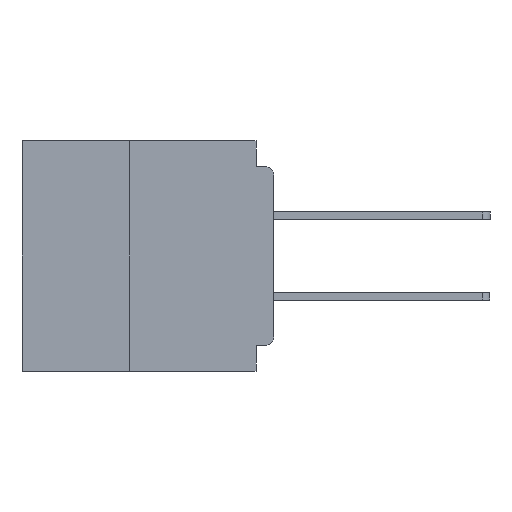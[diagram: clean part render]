
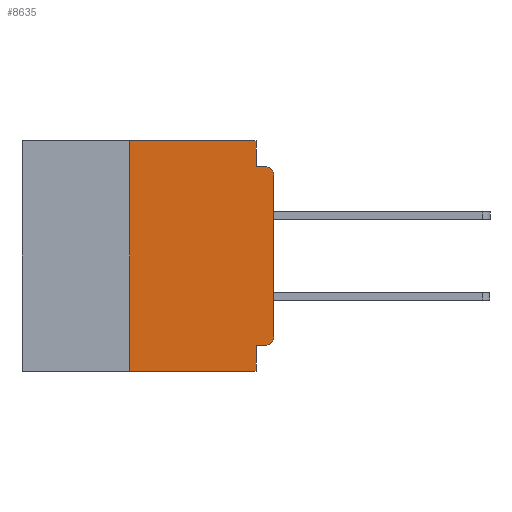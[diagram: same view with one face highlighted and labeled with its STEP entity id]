
A CAD part, left-side view. The second image highlights one B-rep face of the part: STEP entity #8635.
In plain terms, the highlighted planar face has unit normal (-1, 0, 0).
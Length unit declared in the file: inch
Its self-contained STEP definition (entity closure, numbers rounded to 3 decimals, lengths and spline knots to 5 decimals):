
#691 = CARTESIAN_POINT ( 'NONE',  ( 0., 0.031, 0. ) ) ;
#788 = CIRCLE ( 'NONE', #22357, 0.015 ) ;
#1027 = CARTESIAN_POINT ( 'NONE',  ( 0., 0.437, 0. ) ) ;
#2034 = CARTESIAN_POINT ( 'NONE',  ( 0., 0.015, -0.045 ) ) ;
#2985 = EDGE_CURVE ( 'NONE', #43031, #33308, #5848, .T. ) ;
#2990 = LINE ( 'NONE', #50538, #21661 ) ;
#3329 = CARTESIAN_POINT ( 'NONE',  ( 0., 0.015, -0.06 ) ) ;
#5081 = EDGE_CURVE ( 'NONE', #33308, #11062, #788, .T. ) ;
#5328 = EDGE_CURVE ( 'NONE', #40822, #6536, #53416, .T. ) ;
#5631 = VERTEX_POINT ( 'NONE', #53256 ) ;
#5848 = LINE ( 'NONE', #26237, #15844 ) ;
#6536 = VERTEX_POINT ( 'NONE', #42784 ) ;
#7572 = DIRECTION ( 'NONE',  ( 0., 0., -1. ) ) ;
#8548 = ORIENTED_EDGE ( 'NONE', *, *, #28978, .T. ) ;
#8635 = ADVANCED_FACE ( 'NONE', ( #8976 ), #18009, .F. ) ;
#8976 = FACE_OUTER_BOUND ( 'NONE', #48252, .T. ) ;
#9121 = VECTOR ( 'NONE', #34811, 39.37008 ) ;
#9274 = VERTEX_POINT ( 'NONE', #18303 ) ;
#9562 = DIRECTION ( 'NONE',  ( 0., 0., -1. ) ) ;
#10296 = CARTESIAN_POINT ( 'NONE',  ( 0., 0., -0.06 ) ) ;
#11062 = VERTEX_POINT ( 'NONE', #2034 ) ;
#11220 = CARTESIAN_POINT ( 'NONE',  ( 0., 0.437, -0.4 ) ) ;
#12491 = LINE ( 'NONE', #11220, #33768 ) ;
#12582 = LINE ( 'NONE', #50322, #36496 ) ;
#13017 = VECTOR ( 'NONE', #22300, 39.37008 ) ;
#13516 = DIRECTION ( 'NONE',  ( 0., 0., 1. ) ) ;
#15212 = ORIENTED_EDGE ( 'NONE', *, *, #45005, .F. ) ;
#15306 = AXIS2_PLACEMENT_3D ( 'NONE', #1027, #35007, #9562 ) ;
#15700 = LINE ( 'NONE', #43263, #13017 ) ;
#15844 = VECTOR ( 'NONE', #26542, 39.37008 ) ;
#15847 = VERTEX_POINT ( 'NONE', #26275 ) ;
#17436 = VERTEX_POINT ( 'NONE', #44645 ) ;
#18009 = PLANE ( 'NONE',  #15306 ) ;
#18303 = CARTESIAN_POINT ( 'NONE',  ( 0., 0.031, -0.045 ) ) ;
#18527 = CARTESIAN_POINT ( 'NONE',  ( 0., 0.015, -0.34 ) ) ;
#19420 = EDGE_CURVE ( 'NONE', #15847, #17436, #21858, .T. ) ;
#20722 = EDGE_CURVE ( 'NONE', #17436, #5631, #15700, .T. ) ;
#21186 = EDGE_CURVE ( 'NONE', #9274, #11062, #2990, .T. ) ;
#21661 = VECTOR ( 'NONE', #34069, 39.37008 ) ;
#21858 = LINE ( 'NONE', #22060, #9121 ) ;
#21923 = ORIENTED_EDGE ( 'NONE', *, *, #5328, .F. ) ;
#22060 = CARTESIAN_POINT ( 'NONE',  ( 0., 0., -0.355 ) ) ;
#22300 = DIRECTION ( 'NONE',  ( 0., 0., -1. ) ) ;
#22357 = AXIS2_PLACEMENT_3D ( 'NONE', #3329, #33064, #7572 ) ;
#22798 = DIRECTION ( 'NONE',  ( 0., 0., -1. ) ) ;
#25472 = CARTESIAN_POINT ( 'NONE',  ( 0., 0.031, 0. ) ) ;
#25900 = ORIENTED_EDGE ( 'NONE', *, *, #43284, .T. ) ;
#26237 = CARTESIAN_POINT ( 'NONE',  ( 0., 0., 0. ) ) ;
#26275 = CARTESIAN_POINT ( 'NONE',  ( 0., 0.015, -0.355 ) ) ;
#26542 = DIRECTION ( 'NONE',  ( 0., 0., 1. ) ) ;
#28978 = EDGE_CURVE ( 'NONE', #15847, #43031, #40897, .T. ) ;
#29387 = EDGE_CURVE ( 'NONE', #6536, #44907, #12582, .T. ) ;
#30440 = CARTESIAN_POINT ( 'NONE',  ( 0., 0.25, -0.4 ) ) ;
#30451 = DIRECTION ( 'NONE',  ( 0., 0., -1. ) ) ;
#33064 = DIRECTION ( 'NONE',  ( -1., 0., 0. ) ) ;
#33308 = VERTEX_POINT ( 'NONE', #10296 ) ;
#33573 = VECTOR ( 'NONE', #30451, 39.37008 ) ;
#33768 = VECTOR ( 'NONE', #36654, 39.37008 ) ;
#34069 = DIRECTION ( 'NONE',  ( 0., -1., 0. ) ) ;
#34811 = DIRECTION ( 'NONE',  ( 0., 1., 0. ) ) ;
#35007 = DIRECTION ( 'NONE',  ( 1., 0., 0. ) ) ;
#36496 = VECTOR ( 'NONE', #54429, 39.37008 ) ;
#36654 = DIRECTION ( 'NONE',  ( 0., -1., 0. ) ) ;
#40822 = VERTEX_POINT ( 'NONE', #44961 ) ;
#40897 = CIRCLE ( 'NONE', #43734, 0.015 ) ;
#42530 = VECTOR ( 'NONE', #13516, 39.37008 ) ;
#42784 = CARTESIAN_POINT ( 'NONE',  ( 0., 0.25, 0. ) ) ;
#43031 = VERTEX_POINT ( 'NONE', #43425 ) ;
#43263 = CARTESIAN_POINT ( 'NONE',  ( 0., 0.031, -0.4 ) ) ;
#43284 = EDGE_CURVE ( 'NONE', #40822, #5631, #12491, .T. ) ;
#43394 = LINE ( 'NONE', #691, #33573 ) ;
#43425 = CARTESIAN_POINT ( 'NONE',  ( 0., 0., -0.34 ) ) ;
#43734 = AXIS2_PLACEMENT_3D ( 'NONE', #18527, #47845, #22798 ) ;
#44645 = CARTESIAN_POINT ( 'NONE',  ( 0., 0.031, -0.355 ) ) ;
#44885 = ORIENTED_EDGE ( 'NONE', *, *, #5081, .T. ) ;
#44907 = VERTEX_POINT ( 'NONE', #25472 ) ;
#44961 = CARTESIAN_POINT ( 'NONE',  ( 0., 0.25, -0.4 ) ) ;
#45005 = EDGE_CURVE ( 'NONE', #44907, #9274, #43394, .T. ) ;
#47444 = ORIENTED_EDGE ( 'NONE', *, *, #21186, .F. ) ;
#47845 = DIRECTION ( 'NONE',  ( -1., 0., 0. ) ) ;
#48118 = ORIENTED_EDGE ( 'NONE', *, *, #20722, .F. ) ;
#48252 = EDGE_LOOP ( 'NONE', ( #54477, #44885, #47444, #15212, #50020, #21923, #25900, #48118, #49413, #8548 ) ) ;
#49413 = ORIENTED_EDGE ( 'NONE', *, *, #19420, .F. ) ;
#50020 = ORIENTED_EDGE ( 'NONE', *, *, #29387, .F. ) ;
#50322 = CARTESIAN_POINT ( 'NONE',  ( 0., 0.437, 0. ) ) ;
#50538 = CARTESIAN_POINT ( 'NONE',  ( 0., 0., -0.045 ) ) ;
#53256 = CARTESIAN_POINT ( 'NONE',  ( 0., 0.031, -0.4 ) ) ;
#53416 = LINE ( 'NONE', #30440, #42530 ) ;
#54429 = DIRECTION ( 'NONE',  ( 0., -1., 0. ) ) ;
#54477 = ORIENTED_EDGE ( 'NONE', *, *, #2985, .T. ) ;
